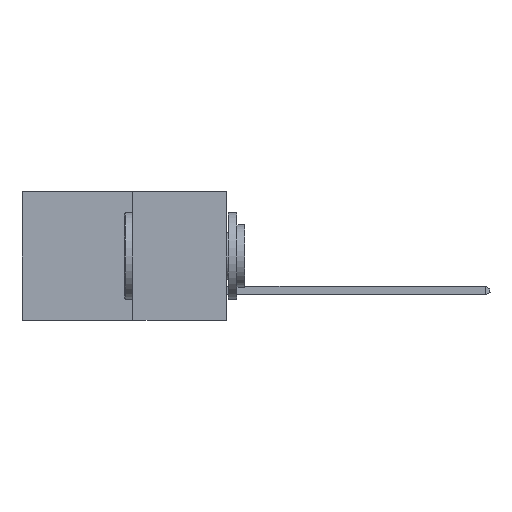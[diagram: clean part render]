
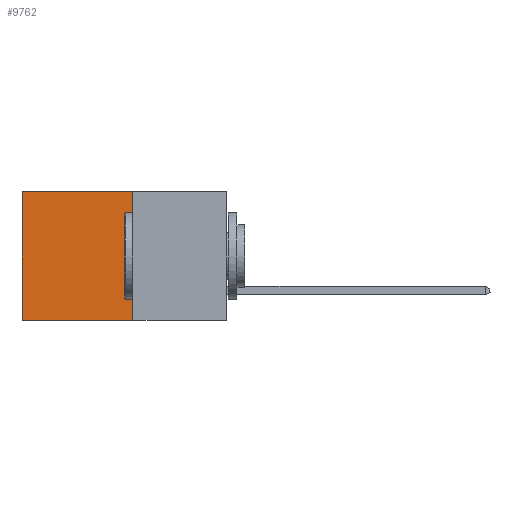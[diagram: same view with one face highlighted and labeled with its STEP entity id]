
A CAD part, left-side view. The second image highlights one B-rep face of the part: STEP entity #9762.
In plain terms, the highlighted planar face has unit normal (-1, 0, 0).
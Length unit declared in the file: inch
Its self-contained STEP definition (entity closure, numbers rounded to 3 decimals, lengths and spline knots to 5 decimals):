
#2188 = LINE ( 'NONE', #18774, #6534 ) ;
#2300 = VERTEX_POINT ( 'NONE', #18981 ) ;
#2307 = AXIS2_PLACEMENT_3D ( 'NONE', #8886, #7135, #20092 ) ;
#2816 = VERTEX_POINT ( 'NONE', #18138 ) ;
#2983 = ORIENTED_EDGE ( 'NONE', *, *, #4495, .F. ) ;
#3997 = CARTESIAN_POINT ( 'NONE',  ( 0.277, 0.27, 0. ) ) ;
#4217 = CARTESIAN_POINT ( 'NONE',  ( 0.277, 0.27, 0. ) ) ;
#4495 = EDGE_CURVE ( 'NONE', #20750, #2300, #13771, .T. ) ;
#6534 = VECTOR ( 'NONE', #16994, 39.37008 ) ;
#7135 = DIRECTION ( 'NONE',  ( 1., 0., 0. ) ) ;
#7725 = CARTESIAN_POINT ( 'NONE',  ( 0.277, 0.59, -0.37 ) ) ;
#8138 = VERTEX_POINT ( 'NONE', #9598 ) ;
#8886 = CARTESIAN_POINT ( 'NONE',  ( 0.277, 0.27, -0.37 ) ) ;
#9541 = EDGE_CURVE ( 'NONE', #20750, #8138, #11224, .T. ) ;
#9598 = CARTESIAN_POINT ( 'NONE',  ( 0.277, 0.59, 0. ) ) ;
#9762 = ADVANCED_FACE ( 'NONE', ( #15867 ), #18226, .F. ) ;
#10441 = ORIENTED_EDGE ( 'NONE', *, *, #9541, .T. ) ;
#11164 = EDGE_LOOP ( 'NONE', ( #22739, #11472, #2983, #10441 ) ) ;
#11224 = LINE ( 'NONE', #4217, #21666 ) ;
#11472 = ORIENTED_EDGE ( 'NONE', *, *, #12631, .F. ) ;
#12227 = LINE ( 'NONE', #7725, #22120 ) ;
#12631 = EDGE_CURVE ( 'NONE', #2300, #2816, #2188, .T. ) ;
#13201 = VECTOR ( 'NONE', #15525, 39.37008 ) ;
#13771 = LINE ( 'NONE', #15639, #13201 ) ;
#15525 = DIRECTION ( 'NONE',  ( 0., 0., -1. ) ) ;
#15639 = CARTESIAN_POINT ( 'NONE',  ( 0.277, 0.27, -0.37 ) ) ;
#15867 = FACE_OUTER_BOUND ( 'NONE', #11164, .T. ) ;
#16994 = DIRECTION ( 'NONE',  ( 0., 1., 0. ) ) ;
#17178 = DIRECTION ( 'NONE',  ( 0., 1., 0. ) ) ;
#17623 = EDGE_CURVE ( 'NONE', #8138, #2816, #12227, .T. ) ;
#18138 = CARTESIAN_POINT ( 'NONE',  ( 0.277, 0.59, -0.37 ) ) ;
#18226 = PLANE ( 'NONE',  #2307 ) ;
#18774 = CARTESIAN_POINT ( 'NONE',  ( 0.277, 0.27, -0.37 ) ) ;
#18981 = CARTESIAN_POINT ( 'NONE',  ( 0.277, 0.27, -0.37 ) ) ;
#20092 = DIRECTION ( 'NONE',  ( 0., 0., -1. ) ) ;
#20699 = DIRECTION ( 'NONE',  ( 0., 0., -1. ) ) ;
#20750 = VERTEX_POINT ( 'NONE', #3997 ) ;
#21666 = VECTOR ( 'NONE', #17178, 39.37008 ) ;
#22120 = VECTOR ( 'NONE', #20699, 39.37008 ) ;
#22739 = ORIENTED_EDGE ( 'NONE', *, *, #17623, .T. ) ;
